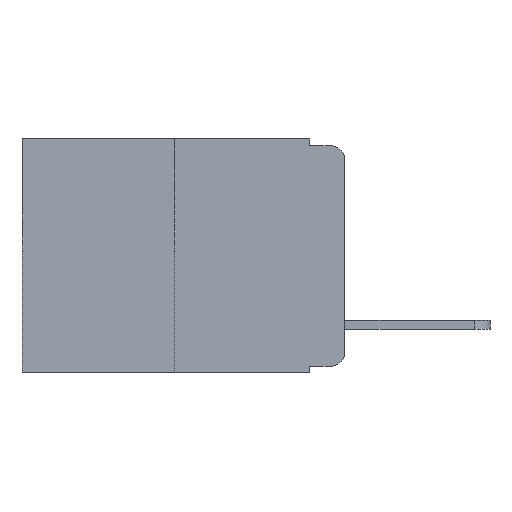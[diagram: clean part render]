
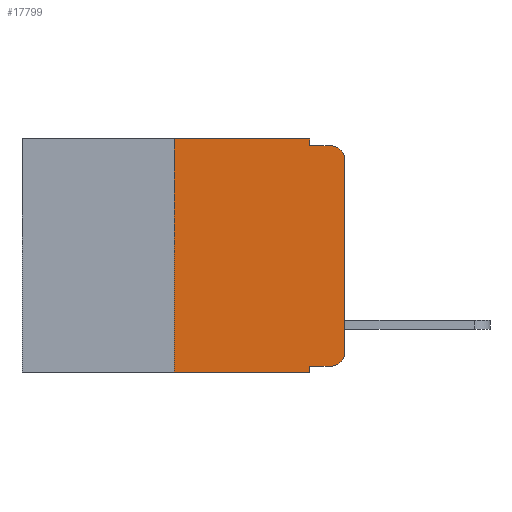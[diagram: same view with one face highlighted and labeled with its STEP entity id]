
A CAD part, left-side view. The second image highlights one B-rep face of the part: STEP entity #17799.
In plain terms, the highlighted planar face has unit normal (-1, 0, 0).
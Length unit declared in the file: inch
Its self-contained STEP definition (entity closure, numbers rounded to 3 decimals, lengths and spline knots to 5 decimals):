
#435 = ORIENTED_EDGE ( 'NONE', *, *, #15572, .T. ) ;
#581 = LINE ( 'NONE', #12560, #17577 ) ;
#653 = VERTEX_POINT ( 'NONE', #7074 ) ;
#692 = DIRECTION ( 'NONE',  ( 0., 0., -1. ) ) ;
#878 = LINE ( 'NONE', #4129, #5167 ) ;
#1070 = CARTESIAN_POINT ( 'NONE',  ( 0., 0.051, 0. ) ) ;
#1376 = PLANE ( 'NONE',  #12528 ) ;
#1430 = EDGE_CURVE ( 'NONE', #11509, #9486, #14423, .T. ) ;
#2141 = CARTESIAN_POINT ( 'NONE',  ( 0., 0.051, -0.343 ) ) ;
#2621 = DIRECTION ( 'NONE',  ( 0., -1., 0. ) ) ;
#2820 = VERTEX_POINT ( 'NONE', #7796 ) ;
#3201 = FACE_OUTER_BOUND ( 'NONE', #4843, .T. ) ;
#3266 = DIRECTION ( 'NONE',  ( 0., -1., 0. ) ) ;
#3560 = DIRECTION ( 'NONE',  ( -1., 0., 0. ) ) ;
#3638 = ORIENTED_EDGE ( 'NONE', *, *, #20849, .F. ) ;
#3955 = LINE ( 'NONE', #8462, #12360 ) ;
#4129 = CARTESIAN_POINT ( 'NONE',  ( 0., 0.051, 0. ) ) ;
#4611 = CARTESIAN_POINT ( 'NONE',  ( 0., 0.02, -0.313 ) ) ;
#4782 = VECTOR ( 'NONE', #12409, 39.37008 ) ;
#4843 = EDGE_LOOP ( 'NONE', ( #15802, #435, #7786, #11783, #14989, #3638, #12328, #9238, #12220, #19640 ) ) ;
#4922 = EDGE_CURVE ( 'NONE', #2820, #16046, #7405, .T. ) ;
#5167 = VECTOR ( 'NONE', #692, 39.37008 ) ;
#6730 = VERTEX_POINT ( 'NONE', #8831 ) ;
#7074 = CARTESIAN_POINT ( 'NONE',  ( 0., 0.051, 0. ) ) ;
#7145 = VECTOR ( 'NONE', #19326, 39.37008 ) ;
#7405 = LINE ( 'NONE', #7979, #7145 ) ;
#7786 = ORIENTED_EDGE ( 'NONE', *, *, #15605, .F. ) ;
#7796 = CARTESIAN_POINT ( 'NONE',  ( 0., 0., -0.313 ) ) ;
#7819 = CARTESIAN_POINT ( 'NONE',  ( 0., 0.25, 0. ) ) ;
#7868 = VECTOR ( 'NONE', #16436, 39.37008 ) ;
#7979 = CARTESIAN_POINT ( 'NONE',  ( 0., 0., 0. ) ) ;
#8146 = VERTEX_POINT ( 'NONE', #7819 ) ;
#8255 = CARTESIAN_POINT ( 'NONE',  ( 0., 0.051, -0.01 ) ) ;
#8462 = CARTESIAN_POINT ( 'NONE',  ( 0., 0.25, 0. ) ) ;
#8546 = VECTOR ( 'NONE', #3266, 39.37008 ) ;
#8831 = CARTESIAN_POINT ( 'NONE',  ( 0., 0.25, -0.343 ) ) ;
#9131 = LINE ( 'NONE', #8255, #7868 ) ;
#9238 = ORIENTED_EDGE ( 'NONE', *, *, #1430, .F. ) ;
#9313 = AXIS2_PLACEMENT_3D ( 'NONE', #4611, #15968, #10791 ) ;
#9455 = LINE ( 'NONE', #11789, #16569 ) ;
#9482 = CARTESIAN_POINT ( 'NONE',  ( 0., 0.051, -0.01 ) ) ;
#9486 = VERTEX_POINT ( 'NONE', #2141 ) ;
#9833 = CARTESIAN_POINT ( 'NONE',  ( 0., 0.02, -0.03 ) ) ;
#10679 = CARTESIAN_POINT ( 'NONE',  ( 0., 0.051, -0.333 ) ) ;
#10791 = DIRECTION ( 'NONE',  ( 0., 0., -1. ) ) ;
#11509 = VERTEX_POINT ( 'NONE', #10679 ) ;
#11663 = DIRECTION ( 'NONE',  ( 0., 0., -1. ) ) ;
#11783 = ORIENTED_EDGE ( 'NONE', *, *, #14150, .F. ) ;
#11789 = CARTESIAN_POINT ( 'NONE',  ( 0., 0.473, 0. ) ) ;
#12144 = LINE ( 'NONE', #19563, #8546 ) ;
#12220 = ORIENTED_EDGE ( 'NONE', *, *, #16796, .T. ) ;
#12328 = ORIENTED_EDGE ( 'NONE', *, *, #14768, .T. ) ;
#12360 = VECTOR ( 'NONE', #16520, 39.37008 ) ;
#12409 = DIRECTION ( 'NONE',  ( 0., 0., -1. ) ) ;
#12528 = AXIS2_PLACEMENT_3D ( 'NONE', #12984, #17739, #14342 ) ;
#12560 = CARTESIAN_POINT ( 'NONE',  ( 0., 0.473, -0.343 ) ) ;
#12805 = VERTEX_POINT ( 'NONE', #16642 ) ;
#12984 = CARTESIAN_POINT ( 'NONE',  ( 0., 0.473, 0. ) ) ;
#13150 = EDGE_CURVE ( 'NONE', #14309, #2820, #18660, .T. ) ;
#14150 = EDGE_CURVE ( 'NONE', #653, #20545, #878, .T. ) ;
#14309 = VERTEX_POINT ( 'NONE', #18448 ) ;
#14334 = EDGE_CURVE ( 'NONE', #8146, #653, #9455, .T. ) ;
#14342 = DIRECTION ( 'NONE',  ( 0., 0., -1. ) ) ;
#14423 = LINE ( 'NONE', #1070, #4782 ) ;
#14768 = EDGE_CURVE ( 'NONE', #6730, #9486, #581, .T. ) ;
#14989 = ORIENTED_EDGE ( 'NONE', *, *, #14334, .F. ) ;
#15196 = DIRECTION ( 'NONE',  ( 0., -1., 0. ) ) ;
#15572 = EDGE_CURVE ( 'NONE', #16046, #12805, #16513, .T. ) ;
#15605 = EDGE_CURVE ( 'NONE', #20545, #12805, #9131, .T. ) ;
#15802 = ORIENTED_EDGE ( 'NONE', *, *, #4922, .T. ) ;
#15968 = DIRECTION ( 'NONE',  ( -1., 0., 0. ) ) ;
#16046 = VERTEX_POINT ( 'NONE', #17824 ) ;
#16436 = DIRECTION ( 'NONE',  ( 0., -1., 0. ) ) ;
#16513 = CIRCLE ( 'NONE', #17925, 0.02 ) ;
#16520 = DIRECTION ( 'NONE',  ( 0., 0., 1. ) ) ;
#16569 = VECTOR ( 'NONE', #15196, 39.37008 ) ;
#16642 = CARTESIAN_POINT ( 'NONE',  ( 0., 0.02, -0.01 ) ) ;
#16796 = EDGE_CURVE ( 'NONE', #11509, #14309, #12144, .T. ) ;
#17577 = VECTOR ( 'NONE', #2621, 39.37008 ) ;
#17739 = DIRECTION ( 'NONE',  ( 1., 0., 0. ) ) ;
#17799 = ADVANCED_FACE ( 'NONE', ( #3201 ), #1376, .F. ) ;
#17824 = CARTESIAN_POINT ( 'NONE',  ( 0., 0., -0.03 ) ) ;
#17925 = AXIS2_PLACEMENT_3D ( 'NONE', #9833, #3560, #11663 ) ;
#18448 = CARTESIAN_POINT ( 'NONE',  ( 0., 0.02, -0.333 ) ) ;
#18660 = CIRCLE ( 'NONE', #9313, 0.02 ) ;
#19326 = DIRECTION ( 'NONE',  ( 0., 0., 1. ) ) ;
#19563 = CARTESIAN_POINT ( 'NONE',  ( 0., 0.051, -0.333 ) ) ;
#19640 = ORIENTED_EDGE ( 'NONE', *, *, #13150, .T. ) ;
#20545 = VERTEX_POINT ( 'NONE', #9482 ) ;
#20849 = EDGE_CURVE ( 'NONE', #6730, #8146, #3955, .T. ) ;
